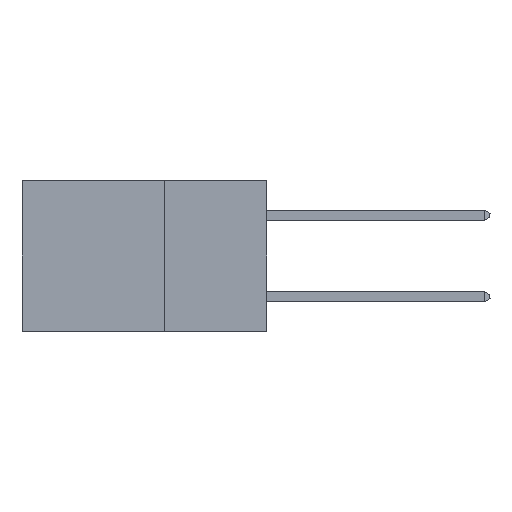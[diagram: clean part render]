
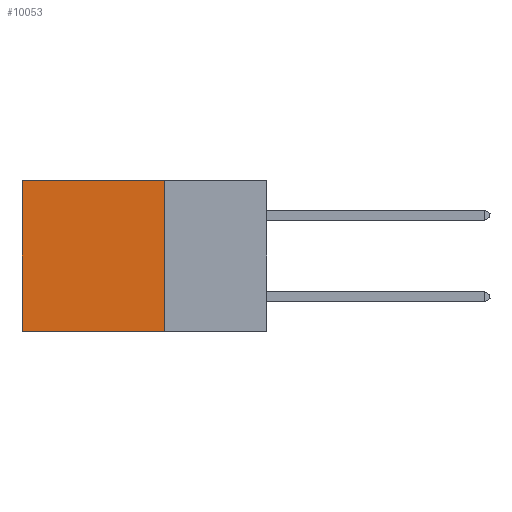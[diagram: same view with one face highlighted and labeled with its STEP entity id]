
A CAD part, left-side view. The second image highlights one B-rep face of the part: STEP entity #10053.
In plain terms, the highlighted planar face has unit normal (-1, 0, 0).
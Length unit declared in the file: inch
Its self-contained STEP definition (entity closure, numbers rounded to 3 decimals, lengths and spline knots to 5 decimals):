
#145 = LINE ( 'NONE', #12408, #5018 ) ;
#318 = CARTESIAN_POINT ( 'NONE',  ( 0.2875, 0.25, -0.37 ) ) ;
#802 = VERTEX_POINT ( 'NONE', #13084 ) ;
#804 = CARTESIAN_POINT ( 'NONE',  ( 0.2875, 0.6, 0. ) ) ;
#893 = LINE ( 'NONE', #12613, #10519 ) ;
#1157 = DIRECTION ( 'NONE',  ( 0., 0., -1. ) ) ;
#1854 = CARTESIAN_POINT ( 'NONE',  ( 0.2875, 0.6, -0.37 ) ) ;
#1945 = EDGE_CURVE ( 'NONE', #802, #10870, #9843, .T. ) ;
#2252 = VECTOR ( 'NONE', #9440, 39.37008 ) ;
#2906 = EDGE_CURVE ( 'NONE', #802, #6297, #893, .T. ) ;
#3264 = CARTESIAN_POINT ( 'NONE',  ( 0.2875, 0.25, 0. ) ) ;
#3925 = VECTOR ( 'NONE', #1157, 39.37008 ) ;
#5018 = VECTOR ( 'NONE', #13346, 39.37008 ) ;
#6046 = AXIS2_PLACEMENT_3D ( 'NONE', #3264, #11436, #7947 ) ;
#6297 = VERTEX_POINT ( 'NONE', #804 ) ;
#6481 = VERTEX_POINT ( 'NONE', #1854 ) ;
#6555 = ORIENTED_EDGE ( 'NONE', *, *, #2906, .T. ) ;
#6598 = PLANE ( 'NONE',  #6046 ) ;
#7081 = EDGE_CURVE ( 'NONE', #6297, #6481, #7999, .T. ) ;
#7947 = DIRECTION ( 'NONE',  ( 0., 0., -1. ) ) ;
#7999 = LINE ( 'NONE', #9493, #2252 ) ;
#9440 = DIRECTION ( 'NONE',  ( 0., 0., -1. ) ) ;
#9493 = CARTESIAN_POINT ( 'NONE',  ( 0.2875, 0.6, 0. ) ) ;
#9819 = DIRECTION ( 'NONE',  ( 0., 1., 0. ) ) ;
#9843 = LINE ( 'NONE', #11976, #3925 ) ;
#10053 = ADVANCED_FACE ( 'NONE', ( #13385 ), #6598, .F. ) ;
#10125 = ORIENTED_EDGE ( 'NONE', *, *, #1945, .F. ) ;
#10519 = VECTOR ( 'NONE', #9819, 39.37008 ) ;
#10870 = VERTEX_POINT ( 'NONE', #318 ) ;
#11168 = ORIENTED_EDGE ( 'NONE', *, *, #12096, .F. ) ;
#11200 = ORIENTED_EDGE ( 'NONE', *, *, #7081, .T. ) ;
#11398 = EDGE_LOOP ( 'NONE', ( #11200, #11168, #10125, #6555 ) ) ;
#11436 = DIRECTION ( 'NONE',  ( 1., 0., 0. ) ) ;
#11976 = CARTESIAN_POINT ( 'NONE',  ( 0.2875, 0.25, 0. ) ) ;
#12096 = EDGE_CURVE ( 'NONE', #10870, #6481, #145, .T. ) ;
#12408 = CARTESIAN_POINT ( 'NONE',  ( 0.2875, 0.25, -0.37 ) ) ;
#12613 = CARTESIAN_POINT ( 'NONE',  ( 0.2875, 0.25, 0. ) ) ;
#13084 = CARTESIAN_POINT ( 'NONE',  ( 0.2875, 0.25, 0. ) ) ;
#13346 = DIRECTION ( 'NONE',  ( 0., 1., 0. ) ) ;
#13385 = FACE_OUTER_BOUND ( 'NONE', #11398, .T. ) ;
